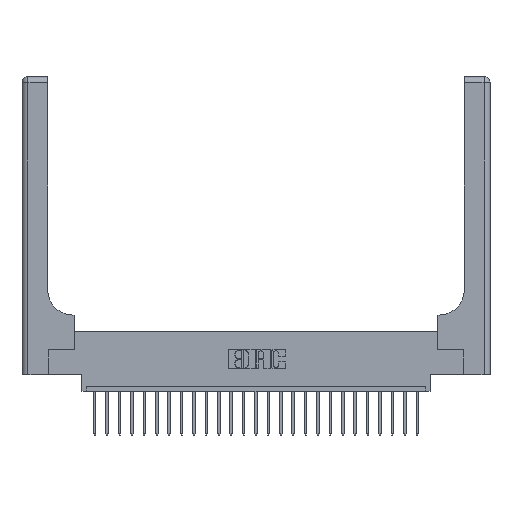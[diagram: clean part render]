
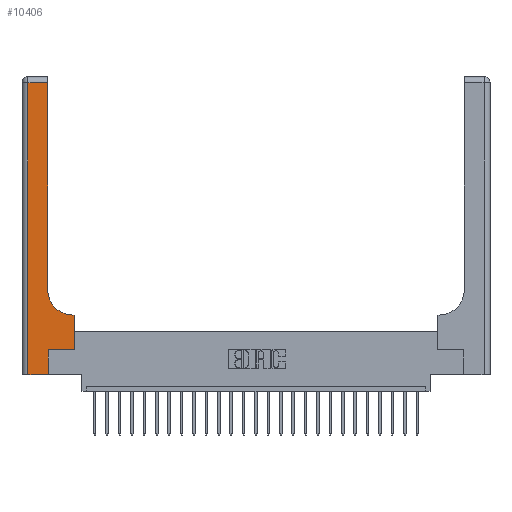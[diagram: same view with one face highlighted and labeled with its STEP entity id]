
A CAD part, top view. The second image highlights one B-rep face of the part: STEP entity #10406.
In plain terms, the highlighted planar face has unit normal (0, 0, 1).
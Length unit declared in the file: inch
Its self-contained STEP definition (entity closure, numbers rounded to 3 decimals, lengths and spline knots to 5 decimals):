
#181 = EDGE_CURVE ( 'NONE', #6085, #3570, #9201, .T. ) ;
#265 = ORIENTED_EDGE ( 'NONE', *, *, #18362, .T. ) ;
#356 = EDGE_LOOP ( 'NONE', ( #14596, #17273, #5011, #265, #24545, #13311, #10097, #17354, #3092 ) ) ;
#366 = LINE ( 'NONE', #13666, #11512 ) ;
#418 = DIRECTION ( 'NONE',  ( 0., 0., -1. ) ) ;
#709 = EDGE_CURVE ( 'NONE', #18458, #8256, #14613, .T. ) ;
#1135 = CARTESIAN_POINT ( 'NONE',  ( 0.26, 0.6, 0.37 ) ) ;
#1745 = LINE ( 'NONE', #2232, #13578 ) ;
#2036 = VERTEX_POINT ( 'NONE', #23580 ) ;
#2221 = DIRECTION ( 'NONE',  ( 0., 1., 0. ) ) ;
#2232 = CARTESIAN_POINT ( 'NONE',  ( 0., 0., 0.37 ) ) ;
#2241 = EDGE_CURVE ( 'NONE', #21852, #6085, #20677, .T. ) ;
#2560 = VECTOR ( 'NONE', #2221, 39.37008 ) ;
#2830 = CARTESIAN_POINT ( 'NONE',  ( 0.06, 2.94, 0.37 ) ) ;
#3092 = ORIENTED_EDGE ( 'NONE', *, *, #21180, .T. ) ;
#3570 = VERTEX_POINT ( 'NONE', #20961 ) ;
#3716 = VECTOR ( 'NONE', #15497, 39.37008 ) ;
#4179 = EDGE_CURVE ( 'NONE', #2036, #18458, #366, .T. ) ;
#5011 = ORIENTED_EDGE ( 'NONE', *, *, #181, .T. ) ;
#5242 = FACE_OUTER_BOUND ( 'NONE', #356, .T. ) ;
#6085 = VERTEX_POINT ( 'NONE', #2830 ) ;
#6128 = DIRECTION ( 'NONE',  ( 1., 0., 0. ) ) ;
#6289 = VERTEX_POINT ( 'NONE', #17330 ) ;
#6834 = DIRECTION ( 'NONE',  ( -1., 0., 0. ) ) ;
#8086 = VERTEX_POINT ( 'NONE', #10015 ) ;
#8256 = VERTEX_POINT ( 'NONE', #18941 ) ;
#9201 = LINE ( 'NONE', #12956, #3716 ) ;
#9331 = VECTOR ( 'NONE', #18811, 39.37008 ) ;
#9549 = DIRECTION ( 'NONE',  ( 0., 1., 0. ) ) ;
#10015 = CARTESIAN_POINT ( 'NONE',  ( 0.26, 0.85, 0.37 ) ) ;
#10097 = ORIENTED_EDGE ( 'NONE', *, *, #20387, .T. ) ;
#10406 = ADVANCED_FACE ( 'NONE', ( #5242 ), #23984, .F. ) ;
#10934 = VECTOR ( 'NONE', #12114, 39.37008 ) ;
#11241 = CARTESIAN_POINT ( 'NONE',  ( 0., 2.94, 0.37 ) ) ;
#11422 = EDGE_CURVE ( 'NONE', #8086, #21852, #17557, .T. ) ;
#11512 = VECTOR ( 'NONE', #9549, 39.37008 ) ;
#12114 = DIRECTION ( 'NONE',  ( 0., 1., 0. ) ) ;
#12864 = DIRECTION ( 'NONE',  ( 1., 0., 0. ) ) ;
#12956 = CARTESIAN_POINT ( 'NONE',  ( 0.06, 3., 0.37 ) ) ;
#13311 = ORIENTED_EDGE ( 'NONE', *, *, #709, .T. ) ;
#13578 = VECTOR ( 'NONE', #22606, 39.37008 ) ;
#13590 = CARTESIAN_POINT ( 'NONE',  ( 0.51, 0.85, 0.37 ) ) ;
#13666 = CARTESIAN_POINT ( 'NONE',  ( 0.265, 0., 0.37 ) ) ;
#13915 = VECTOR ( 'NONE', #12864, 39.37008 ) ;
#14596 = ORIENTED_EDGE ( 'NONE', *, *, #11422, .T. ) ;
#14613 = LINE ( 'NONE', #14733, #13915 ) ;
#14733 = CARTESIAN_POINT ( 'NONE',  ( 0.265, 0.25, 0.37 ) ) ;
#15496 = LINE ( 'NONE', #19098, #2560 ) ;
#15497 = DIRECTION ( 'NONE',  ( 0., -1., 0. ) ) ;
#15653 = CARTESIAN_POINT ( 'NONE',  ( 0.528, 0.6, 0.37 ) ) ;
#16826 = AXIS2_PLACEMENT_3D ( 'NONE', #13590, #418, #6128 ) ;
#17273 = ORIENTED_EDGE ( 'NONE', *, *, #2241, .T. ) ;
#17330 = CARTESIAN_POINT ( 'NONE',  ( 0.51, 0.6, 0.37 ) ) ;
#17354 = ORIENTED_EDGE ( 'NONE', *, *, #20169, .T. ) ;
#17557 = LINE ( 'NONE', #23153, #10934 ) ;
#17583 = CARTESIAN_POINT ( 'NONE',  ( 0.26, 2.94, 0.37 ) ) ;
#17861 = CARTESIAN_POINT ( 'NONE',  ( 0.265, 0.25, 0.37 ) ) ;
#18029 = DIRECTION ( 'NONE',  ( 0., 0., -1. ) ) ;
#18154 = DIRECTION ( 'NONE',  ( -1., 0., 0. ) ) ;
#18362 = EDGE_CURVE ( 'NONE', #3570, #2036, #1745, .T. ) ;
#18458 = VERTEX_POINT ( 'NONE', #17861 ) ;
#18811 = DIRECTION ( 'NONE',  ( -1., 0., 0. ) ) ;
#18941 = CARTESIAN_POINT ( 'NONE',  ( 0.528, 0.25, 0.37 ) ) ;
#19098 = CARTESIAN_POINT ( 'NONE',  ( 0.528, 0.25, 0.37 ) ) ;
#19893 = CARTESIAN_POINT ( 'NONE',  ( 0., 3., 0.37 ) ) ;
#20035 = VERTEX_POINT ( 'NONE', #15653 ) ;
#20169 = EDGE_CURVE ( 'NONE', #20035, #6289, #22120, .T. ) ;
#20387 = EDGE_CURVE ( 'NONE', #8256, #20035, #15496, .T. ) ;
#20399 = AXIS2_PLACEMENT_3D ( 'NONE', #19893, #18029, #18154 ) ;
#20677 = LINE ( 'NONE', #11241, #9331 ) ;
#20961 = CARTESIAN_POINT ( 'NONE',  ( 0.06, 0., 0.37 ) ) ;
#21180 = EDGE_CURVE ( 'NONE', #6289, #8086, #23972, .T. ) ;
#21852 = VERTEX_POINT ( 'NONE', #17583 ) ;
#22120 = LINE ( 'NONE', #1135, #24325 ) ;
#22606 = DIRECTION ( 'NONE',  ( 1., 0., 0. ) ) ;
#23153 = CARTESIAN_POINT ( 'NONE',  ( 0.26, 3., 0.37 ) ) ;
#23580 = CARTESIAN_POINT ( 'NONE',  ( 0.265, 0., 0.37 ) ) ;
#23972 = CIRCLE ( 'NONE', #16826, 0.25 ) ;
#23984 = PLANE ( 'NONE',  #20399 ) ;
#24325 = VECTOR ( 'NONE', #6834, 39.37008 ) ;
#24545 = ORIENTED_EDGE ( 'NONE', *, *, #4179, .T. ) ;
